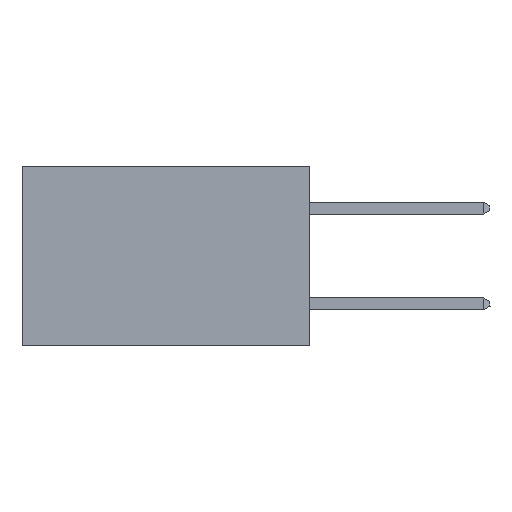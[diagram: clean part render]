
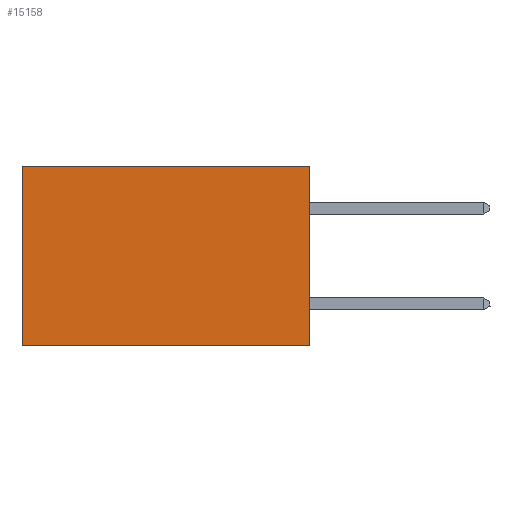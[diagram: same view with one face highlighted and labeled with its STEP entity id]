
A CAD part, left-side view. The second image highlights one B-rep face of the part: STEP entity #15158.
In plain terms, the highlighted planar face has unit normal (-1, 0, 0).
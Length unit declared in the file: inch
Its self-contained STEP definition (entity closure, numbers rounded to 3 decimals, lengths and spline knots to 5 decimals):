
#800 = DIRECTION ( 'NONE',  ( 0., 0., -1. ) ) ;
#1260 = VERTEX_POINT ( 'NONE', #19158 ) ;
#1418 = EDGE_CURVE ( 'NONE', #1260, #10759, #2432, .T. ) ;
#2432 = LINE ( 'NONE', #13105, #17873 ) ;
#2788 = LINE ( 'NONE', #9013, #15344 ) ;
#2820 = ORIENTED_EDGE ( 'NONE', *, *, #1418, .F. ) ;
#4875 = DIRECTION ( 'NONE',  ( 0., 1., 0. ) ) ;
#5493 = CARTESIAN_POINT ( 'NONE',  ( 0.2875, 0., -0.375 ) ) ;
#5524 = VECTOR ( 'NONE', #10162, 39.37008 ) ;
#6540 = CARTESIAN_POINT ( 'NONE',  ( 0.2875, 0., 0. ) ) ;
#6555 = PLANE ( 'NONE',  #20498 ) ;
#7472 = EDGE_CURVE ( 'NONE', #1260, #19823, #20751, .T. ) ;
#8246 = CARTESIAN_POINT ( 'NONE',  ( 0.2875, 0., -0.375 ) ) ;
#9013 = CARTESIAN_POINT ( 'NONE',  ( 0.2875, 0.6, -0.375 ) ) ;
#9786 = VERTEX_POINT ( 'NONE', #18048 ) ;
#9862 = CARTESIAN_POINT ( 'NONE',  ( 0.2875, 0., -0.375 ) ) ;
#9915 = CARTESIAN_POINT ( 'NONE',  ( 0.2875, 0.6, 0. ) ) ;
#9961 = DIRECTION ( 'NONE',  ( 0., 0., -1. ) ) ;
#10162 = DIRECTION ( 'NONE',  ( 0., 1., 0. ) ) ;
#10759 = VERTEX_POINT ( 'NONE', #5493 ) ;
#12682 = FACE_OUTER_BOUND ( 'NONE', #14212, .T. ) ;
#13029 = LINE ( 'NONE', #9862, #20913 ) ;
#13105 = CARTESIAN_POINT ( 'NONE',  ( 0.2875, 0., -0.375 ) ) ;
#13364 = ORIENTED_EDGE ( 'NONE', *, *, #20244, .T. ) ;
#14132 = ORIENTED_EDGE ( 'NONE', *, *, #7472, .T. ) ;
#14212 = EDGE_LOOP ( 'NONE', ( #13364, #17204, #2820, #14132 ) ) ;
#15158 = ADVANCED_FACE ( 'NONE', ( #12682 ), #6555, .F. ) ;
#15344 = VECTOR ( 'NONE', #800, 39.37008 ) ;
#16405 = DIRECTION ( 'NONE',  ( 1., 0., 0. ) ) ;
#17204 = ORIENTED_EDGE ( 'NONE', *, *, #19139, .F. ) ;
#17873 = VECTOR ( 'NONE', #19987, 39.37008 ) ;
#18048 = CARTESIAN_POINT ( 'NONE',  ( 0.2875, 0.6, -0.375 ) ) ;
#19139 = EDGE_CURVE ( 'NONE', #10759, #9786, #13029, .T. ) ;
#19158 = CARTESIAN_POINT ( 'NONE',  ( 0.2875, 0., 0. ) ) ;
#19823 = VERTEX_POINT ( 'NONE', #9915 ) ;
#19987 = DIRECTION ( 'NONE',  ( 0., 0., -1. ) ) ;
#20244 = EDGE_CURVE ( 'NONE', #19823, #9786, #2788, .T. ) ;
#20498 = AXIS2_PLACEMENT_3D ( 'NONE', #8246, #16405, #9961 ) ;
#20751 = LINE ( 'NONE', #6540, #5524 ) ;
#20913 = VECTOR ( 'NONE', #4875, 39.37008 ) ;
